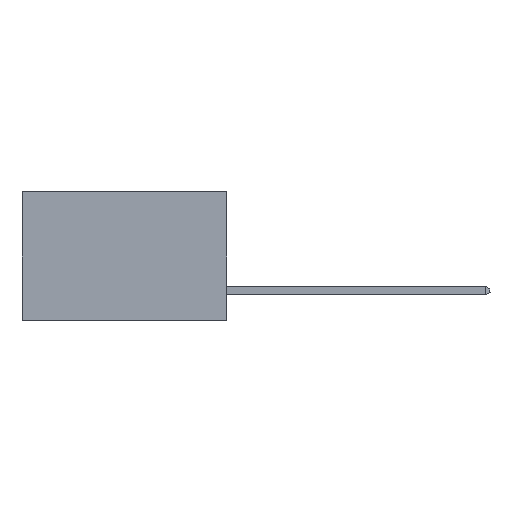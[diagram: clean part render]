
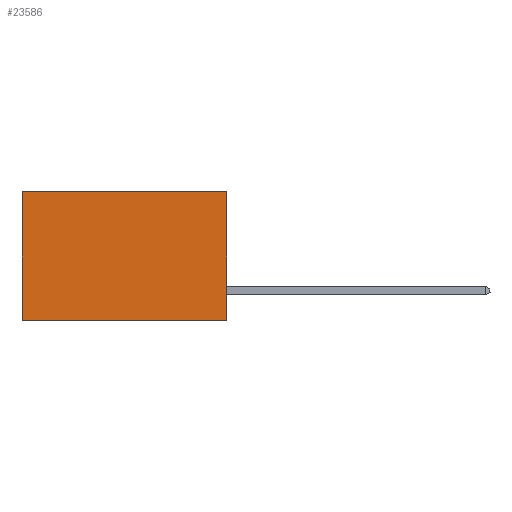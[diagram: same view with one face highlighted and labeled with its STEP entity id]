
A CAD part, left-side view. The second image highlights one B-rep face of the part: STEP entity #23586.
In plain terms, the highlighted planar face has unit normal (-1, 0, 0).
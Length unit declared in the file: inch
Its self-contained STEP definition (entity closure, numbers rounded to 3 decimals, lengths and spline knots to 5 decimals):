
#309 = CARTESIAN_POINT ( 'NONE',  ( 0.277, 0., -0.37 ) ) ;
#507 = CARTESIAN_POINT ( 'NONE',  ( 0.277, 0.59, 0. ) ) ;
#1822 = VECTOR ( 'NONE', #24204, 39.37008 ) ;
#2997 = CARTESIAN_POINT ( 'NONE',  ( 0.277, 0., 0. ) ) ;
#3832 = LINE ( 'NONE', #18731, #24318 ) ;
#4453 = LINE ( 'NONE', #15835, #24881 ) ;
#5142 = FACE_OUTER_BOUND ( 'NONE', #25668, .T. ) ;
#5562 = CARTESIAN_POINT ( 'NONE',  ( 0.277, 0., -0.37 ) ) ;
#6439 = VERTEX_POINT ( 'NONE', #8674 ) ;
#6626 = CARTESIAN_POINT ( 'NONE',  ( 0.277, 0., 0. ) ) ;
#6656 = AXIS2_PLACEMENT_3D ( 'NONE', #5562, #7570, #21502 ) ;
#7222 = LINE ( 'NONE', #309, #1822 ) ;
#7570 = DIRECTION ( 'NONE',  ( 1., 0., 0. ) ) ;
#8410 = ORIENTED_EDGE ( 'NONE', *, *, #24350, .T. ) ;
#8650 = VERTEX_POINT ( 'NONE', #23063 ) ;
#8674 = CARTESIAN_POINT ( 'NONE',  ( 0.277, 0.59, -0.37 ) ) ;
#9903 = DIRECTION ( 'NONE',  ( 0., 0., -1. ) ) ;
#12432 = VERTEX_POINT ( 'NONE', #507 ) ;
#12907 = LINE ( 'NONE', #2997, #17599 ) ;
#14783 = DIRECTION ( 'NONE',  ( 0., 0., -1. ) ) ;
#15835 = CARTESIAN_POINT ( 'NONE',  ( 0.277, 0.59, -0.37 ) ) ;
#17529 = PLANE ( 'NONE',  #6656 ) ;
#17599 = VECTOR ( 'NONE', #19048, 39.37008 ) ;
#18113 = EDGE_CURVE ( 'NONE', #8650, #6439, #7222, .T. ) ;
#18731 = CARTESIAN_POINT ( 'NONE',  ( 0.277, 0., -0.37 ) ) ;
#19048 = DIRECTION ( 'NONE',  ( 0., 1., 0. ) ) ;
#21293 = ORIENTED_EDGE ( 'NONE', *, *, #24649, .T. ) ;
#21502 = DIRECTION ( 'NONE',  ( 0., 0., -1. ) ) ;
#21986 = ORIENTED_EDGE ( 'NONE', *, *, #24002, .F. ) ;
#23063 = CARTESIAN_POINT ( 'NONE',  ( 0.277, 0., -0.37 ) ) ;
#23103 = ORIENTED_EDGE ( 'NONE', *, *, #18113, .F. ) ;
#23586 = ADVANCED_FACE ( 'NONE', ( #5142 ), #17529, .F. ) ;
#24002 = EDGE_CURVE ( 'NONE', #24804, #8650, #3832, .T. ) ;
#24204 = DIRECTION ( 'NONE',  ( 0., 1., 0. ) ) ;
#24318 = VECTOR ( 'NONE', #14783, 39.37008 ) ;
#24350 = EDGE_CURVE ( 'NONE', #12432, #6439, #4453, .T. ) ;
#24649 = EDGE_CURVE ( 'NONE', #24804, #12432, #12907, .T. ) ;
#24804 = VERTEX_POINT ( 'NONE', #6626 ) ;
#24881 = VECTOR ( 'NONE', #9903, 39.37008 ) ;
#25668 = EDGE_LOOP ( 'NONE', ( #8410, #23103, #21986, #21293 ) ) ;
